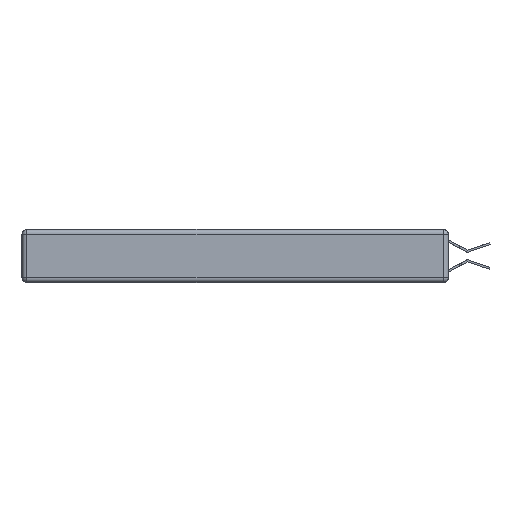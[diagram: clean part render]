
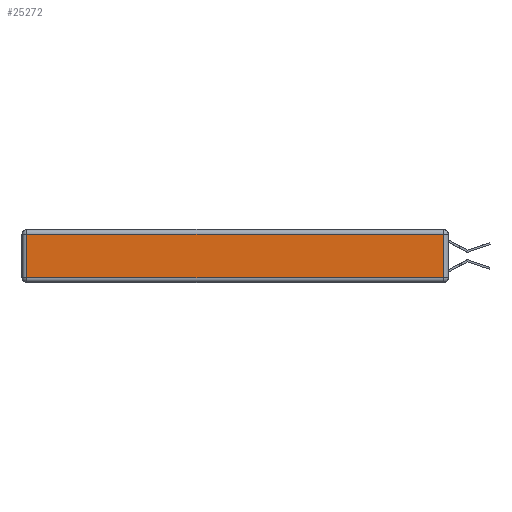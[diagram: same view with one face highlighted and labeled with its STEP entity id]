
A CAD part, left-side view. The second image highlights one B-rep face of the part: STEP entity #25272.
In plain terms, the highlighted planar face has unit normal (-1, 0, 0).
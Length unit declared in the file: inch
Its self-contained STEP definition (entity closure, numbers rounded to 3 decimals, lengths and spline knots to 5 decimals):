
#1526 = CARTESIAN_POINT ( 'NONE',  ( 0., 2.75, -0.03 ) ) ;
#1790 = DIRECTION ( 'NONE',  ( -1., 0., 0. ) ) ;
#2794 = VERTEX_POINT ( 'NONE', #19590 ) ;
#3202 = CARTESIAN_POINT ( 'NONE',  ( 0., 0.03, -0.313 ) ) ;
#3580 = CARTESIAN_POINT ( 'NONE',  ( 0., 0., -0.343 ) ) ;
#3752 = DIRECTION ( 'NONE',  ( 0., 0., 1. ) ) ;
#4725 = CARTESIAN_POINT ( 'NONE',  ( 0., 0., -0.313 ) ) ;
#6015 = FACE_OUTER_BOUND ( 'NONE', #8845, .T. ) ;
#6343 = LINE ( 'NONE', #25186, #16767 ) ;
#6831 = EDGE_CURVE ( 'NONE', #2794, #11746, #12066, .T. ) ;
#8605 = VECTOR ( 'NONE', #20289, 39.37008 ) ;
#8845 = EDGE_LOOP ( 'NONE', ( #23906, #18936, #9446, #9780 ) ) ;
#9446 = ORIENTED_EDGE ( 'NONE', *, *, #13712, .T. ) ;
#9780 = ORIENTED_EDGE ( 'NONE', *, *, #6831, .T. ) ;
#9821 = CARTESIAN_POINT ( 'NONE',  ( 0., 2.72, -0.343 ) ) ;
#10768 = EDGE_CURVE ( 'NONE', #11746, #14750, #13812, .T. ) ;
#11746 = VERTEX_POINT ( 'NONE', #23535 ) ;
#12029 = DIRECTION ( 'NONE',  ( 0., 0., -1. ) ) ;
#12066 = LINE ( 'NONE', #9821, #15445 ) ;
#13019 = DIRECTION ( 'NONE',  ( 0., 1., 0. ) ) ;
#13712 = EDGE_CURVE ( 'NONE', #23036, #2794, #19205, .T. ) ;
#13812 = LINE ( 'NONE', #4725, #8605 ) ;
#14750 = VERTEX_POINT ( 'NONE', #3202 ) ;
#15445 = VECTOR ( 'NONE', #12029, 39.37008 ) ;
#16767 = VECTOR ( 'NONE', #17562, 39.37008 ) ;
#17562 = DIRECTION ( 'NONE',  ( 0., 0., 1. ) ) ;
#18936 = ORIENTED_EDGE ( 'NONE', *, *, #24362, .T. ) ;
#19205 = LINE ( 'NONE', #1526, #24371 ) ;
#19590 = CARTESIAN_POINT ( 'NONE',  ( 0., 2.72, -0.03 ) ) ;
#20289 = DIRECTION ( 'NONE',  ( 0., -1., 0. ) ) ;
#20413 = AXIS2_PLACEMENT_3D ( 'NONE', #3580, #1790, #3752 ) ;
#21414 = PLANE ( 'NONE',  #20413 ) ;
#21964 = CARTESIAN_POINT ( 'NONE',  ( 0., 0.03, -0.03 ) ) ;
#23036 = VERTEX_POINT ( 'NONE', #21964 ) ;
#23535 = CARTESIAN_POINT ( 'NONE',  ( 0., 2.72, -0.313 ) ) ;
#23906 = ORIENTED_EDGE ( 'NONE', *, *, #10768, .T. ) ;
#24362 = EDGE_CURVE ( 'NONE', #14750, #23036, #6343, .T. ) ;
#24371 = VECTOR ( 'NONE', #13019, 39.37008 ) ;
#25186 = CARTESIAN_POINT ( 'NONE',  ( 0., 0.03, -0.343 ) ) ;
#25272 = ADVANCED_FACE ( 'NONE', ( #6015 ), #21414, .T. ) ;
